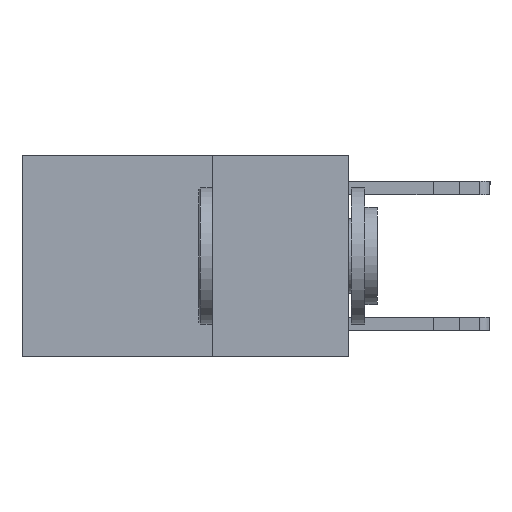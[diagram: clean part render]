
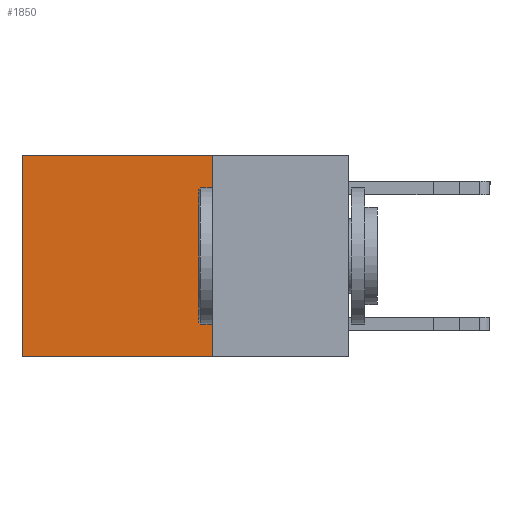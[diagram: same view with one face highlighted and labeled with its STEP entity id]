
A CAD part, left-side view. The second image highlights one B-rep face of the part: STEP entity #1850.
In plain terms, the highlighted planar face has unit normal (-1, 0, 0).
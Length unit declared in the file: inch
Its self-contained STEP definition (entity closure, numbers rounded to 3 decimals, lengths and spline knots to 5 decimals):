
#1191 = DIRECTION ( 'NONE',  ( 0., 0., -1. ) ) ;
#1280 = PLANE ( 'NONE',  #15798 ) ;
#1850 = ADVANCED_FACE ( 'NONE', ( #7096 ), #1280, .F. ) ;
#3054 = CARTESIAN_POINT ( 'NONE',  ( 0.2625, 0.6, 0. ) ) ;
#3469 = CARTESIAN_POINT ( 'NONE',  ( 0.2625, 0.25, 0. ) ) ;
#3630 = DIRECTION ( 'NONE',  ( 0., 1., 0. ) ) ;
#4117 = DIRECTION ( 'NONE',  ( 1., 0., 0. ) ) ;
#4205 = VECTOR ( 'NONE', #14947, 39.37008 ) ;
#5670 = VERTEX_POINT ( 'NONE', #3054 ) ;
#5675 = LINE ( 'NONE', #3469, #4205 ) ;
#5826 = ORIENTED_EDGE ( 'NONE', *, *, #7770, .T. ) ;
#6645 = LINE ( 'NONE', #11006, #16713 ) ;
#7000 = EDGE_LOOP ( 'NONE', ( #5826, #10687, #17481, #25032 ) ) ;
#7057 = CARTESIAN_POINT ( 'NONE',  ( 0.2625, 0.25, -0.37 ) ) ;
#7096 = FACE_OUTER_BOUND ( 'NONE', #7000, .T. ) ;
#7770 = EDGE_CURVE ( 'NONE', #5670, #10686, #10747, .T. ) ;
#8840 = DIRECTION ( 'NONE',  ( 0., 0., -1. ) ) ;
#9253 = EDGE_CURVE ( 'NONE', #13582, #10686, #15491, .T. ) ;
#10686 = VERTEX_POINT ( 'NONE', #15435 ) ;
#10687 = ORIENTED_EDGE ( 'NONE', *, *, #9253, .F. ) ;
#10747 = LINE ( 'NONE', #14858, #19270 ) ;
#11006 = CARTESIAN_POINT ( 'NONE',  ( 0.2625, 0.25, 0. ) ) ;
#13425 = CARTESIAN_POINT ( 'NONE',  ( 0.2625, 0.25, -0.37 ) ) ;
#13582 = VERTEX_POINT ( 'NONE', #7057 ) ;
#14858 = CARTESIAN_POINT ( 'NONE',  ( 0.2625, 0.6, 0. ) ) ;
#14947 = DIRECTION ( 'NONE',  ( 0., 1., 0. ) ) ;
#15435 = CARTESIAN_POINT ( 'NONE',  ( 0.2625, 0.6, -0.37 ) ) ;
#15491 = LINE ( 'NONE', #13425, #20916 ) ;
#15798 = AXIS2_PLACEMENT_3D ( 'NONE', #24843, #4117, #17530 ) ;
#16713 = VECTOR ( 'NONE', #8840, 39.37008 ) ;
#17481 = ORIENTED_EDGE ( 'NONE', *, *, #25197, .F. ) ;
#17530 = DIRECTION ( 'NONE',  ( 0., 0., -1. ) ) ;
#19270 = VECTOR ( 'NONE', #1191, 39.37008 ) ;
#20259 = EDGE_CURVE ( 'NONE', #20523, #5670, #5675, .T. ) ;
#20523 = VERTEX_POINT ( 'NONE', #24447 ) ;
#20916 = VECTOR ( 'NONE', #3630, 39.37008 ) ;
#24447 = CARTESIAN_POINT ( 'NONE',  ( 0.2625, 0.25, 0. ) ) ;
#24843 = CARTESIAN_POINT ( 'NONE',  ( 0.2625, 0.25, 0. ) ) ;
#25032 = ORIENTED_EDGE ( 'NONE', *, *, #20259, .T. ) ;
#25197 = EDGE_CURVE ( 'NONE', #20523, #13582, #6645, .T. ) ;
